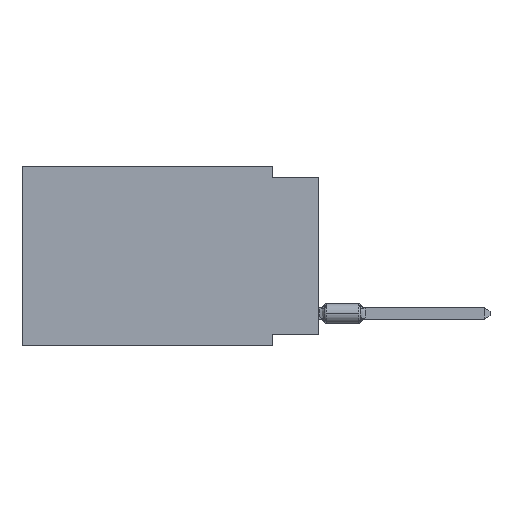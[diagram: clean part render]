
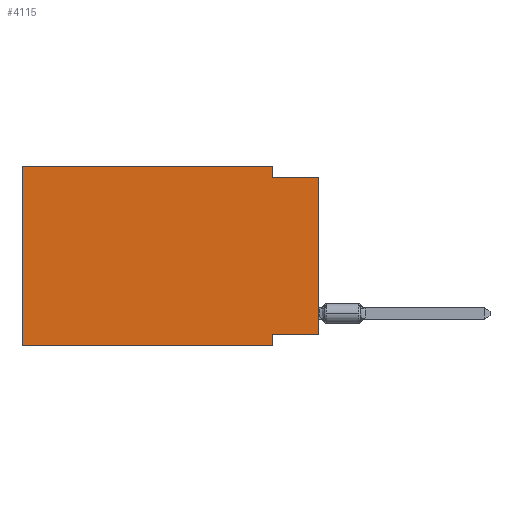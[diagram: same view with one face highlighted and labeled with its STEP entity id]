
A CAD part, left-side view. The second image highlights one B-rep face of the part: STEP entity #4115.
In plain terms, the highlighted planar face has unit normal (-1, 0, 0).
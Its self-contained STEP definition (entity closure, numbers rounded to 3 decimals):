
#9 = EDGE_LOOP ( 'NONE', ( #517, #12821, #6017, #6920, #6965, #12620, #5127, #501 ) ) ;
#72 = LINE ( 'NONE', #10247, #2785 ) ;
#79 = CARTESIAN_POINT ( 'NONE',  ( 0., 2.54, -9.906 ) ) ;
#501 = ORIENTED_EDGE ( 'NONE', *, *, #16031, .F. ) ;
#517 = ORIENTED_EDGE ( 'NONE', *, *, #2343, .T. ) ;
#793 = VERTEX_POINT ( 'NONE', #10577 ) ;
#906 = CARTESIAN_POINT ( 'NONE',  ( 0., 0., 0. ) ) ;
#985 = DIRECTION ( 'NONE',  ( 0., 0., 1. ) ) ;
#1055 = LINE ( 'NONE', #7648, #1431 ) ;
#1083 = LINE ( 'NONE', #11263, #10426 ) ;
#1355 = DIRECTION ( 'NONE',  ( 0., -1., 0. ) ) ;
#1431 = VECTOR ( 'NONE', #10043, 1000. ) ;
#1953 = CARTESIAN_POINT ( 'NONE',  ( 0., 0., -9.271 ) ) ;
#2343 = EDGE_CURVE ( 'NONE', #4718, #3346, #3307, .T. ) ;
#2713 = LINE ( 'NONE', #12883, #4289 ) ;
#2785 = VECTOR ( 'NONE', #10329, 1000. ) ;
#2854 = CARTESIAN_POINT ( 'NONE',  ( 0., 0., -0.635 ) ) ;
#3307 = LINE ( 'NONE', #906, #10120 ) ;
#3317 = LINE ( 'NONE', #1953, #14195 ) ;
#3346 = VERTEX_POINT ( 'NONE', #2854 ) ;
#3515 = CARTESIAN_POINT ( 'NONE',  ( 0., 16.383, 0. ) ) ;
#4088 = VERTEX_POINT ( 'NONE', #3515 ) ;
#4115 = ADVANCED_FACE ( 'NONE', ( #11135 ), #8650, .F. ) ;
#4289 = VECTOR ( 'NONE', #8965, 1000. ) ;
#4718 = VERTEX_POINT ( 'NONE', #15454 ) ;
#4942 = VERTEX_POINT ( 'NONE', #9130 ) ;
#5127 = ORIENTED_EDGE ( 'NONE', *, *, #12560, .F. ) ;
#6017 = ORIENTED_EDGE ( 'NONE', *, *, #14637, .F. ) ;
#6920 = ORIENTED_EDGE ( 'NONE', *, *, #7948, .F. ) ;
#6965 = ORIENTED_EDGE ( 'NONE', *, *, #7162, .F. ) ;
#7162 = EDGE_CURVE ( 'NONE', #793, #4088, #1083, .T. ) ;
#7252 = DIRECTION ( 'NONE',  ( 0., 1., 0. ) ) ;
#7365 = LINE ( 'NONE', #13838, #7412 ) ;
#7412 = VECTOR ( 'NONE', #12555, 1000. ) ;
#7509 = DIRECTION ( 'NONE',  ( 0., 0., 1. ) ) ;
#7648 = CARTESIAN_POINT ( 'NONE',  ( 0., 0., -0.635 ) ) ;
#7948 = EDGE_CURVE ( 'NONE', #4088, #14120, #7365, .T. ) ;
#8617 = CARTESIAN_POINT ( 'NONE',  ( 0., 2.54, 0. ) ) ;
#8650 = PLANE ( 'NONE',  #12929 ) ;
#8965 = DIRECTION ( 'NONE',  ( 0., 0., -1. ) ) ;
#9130 = CARTESIAN_POINT ( 'NONE',  ( 0., 2.54, -9.271 ) ) ;
#9305 = CARTESIAN_POINT ( 'NONE',  ( 0., 16.383, -9.906 ) ) ;
#10043 = DIRECTION ( 'NONE',  ( 0., -1., 0. ) ) ;
#10120 = VECTOR ( 'NONE', #985, 1000. ) ;
#10247 = CARTESIAN_POINT ( 'NONE',  ( 0., 2.54, 0. ) ) ;
#10329 = DIRECTION ( 'NONE',  ( 0., 0., -1. ) ) ;
#10426 = VECTOR ( 'NONE', #7509, 1000. ) ;
#10577 = CARTESIAN_POINT ( 'NONE',  ( 0., 16.383, -9.906 ) ) ;
#11135 = FACE_OUTER_BOUND ( 'NONE', #9, .T. ) ;
#11180 = EDGE_CURVE ( 'NONE', #14373, #3346, #1055, .T. ) ;
#11263 = CARTESIAN_POINT ( 'NONE',  ( 0., 16.383, 0. ) ) ;
#11894 = EDGE_CURVE ( 'NONE', #793, #12556, #15802, .T. ) ;
#12488 = CARTESIAN_POINT ( 'NONE',  ( 0., 2.54, -0.635 ) ) ;
#12555 = DIRECTION ( 'NONE',  ( 0., -1., 0. ) ) ;
#12556 = VERTEX_POINT ( 'NONE', #79 ) ;
#12560 = EDGE_CURVE ( 'NONE', #4942, #12556, #2713, .T. ) ;
#12562 = DIRECTION ( 'NONE',  ( 0., 0., -1. ) ) ;
#12620 = ORIENTED_EDGE ( 'NONE', *, *, #11894, .T. ) ;
#12821 = ORIENTED_EDGE ( 'NONE', *, *, #11180, .F. ) ;
#12883 = CARTESIAN_POINT ( 'NONE',  ( 0., 2.54, -9.906 ) ) ;
#12929 = AXIS2_PLACEMENT_3D ( 'NONE', #15222, #16354, #12562 ) ;
#13190 = VECTOR ( 'NONE', #1355, 1000. ) ;
#13838 = CARTESIAN_POINT ( 'NONE',  ( 0., 16.383, 0. ) ) ;
#14120 = VERTEX_POINT ( 'NONE', #8617 ) ;
#14195 = VECTOR ( 'NONE', #7252, 1000. ) ;
#14373 = VERTEX_POINT ( 'NONE', #12488 ) ;
#14637 = EDGE_CURVE ( 'NONE', #14120, #14373, #72, .T. ) ;
#15222 = CARTESIAN_POINT ( 'NONE',  ( 0., 16.383, 0. ) ) ;
#15454 = CARTESIAN_POINT ( 'NONE',  ( 0., 0., -9.271 ) ) ;
#15802 = LINE ( 'NONE', #9305, #13190 ) ;
#16031 = EDGE_CURVE ( 'NONE', #4718, #4942, #3317, .T. ) ;
#16354 = DIRECTION ( 'NONE',  ( 1., 0., 0. ) ) ;
